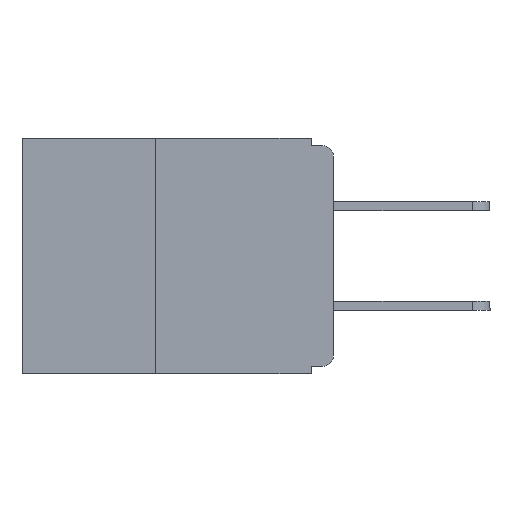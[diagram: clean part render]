
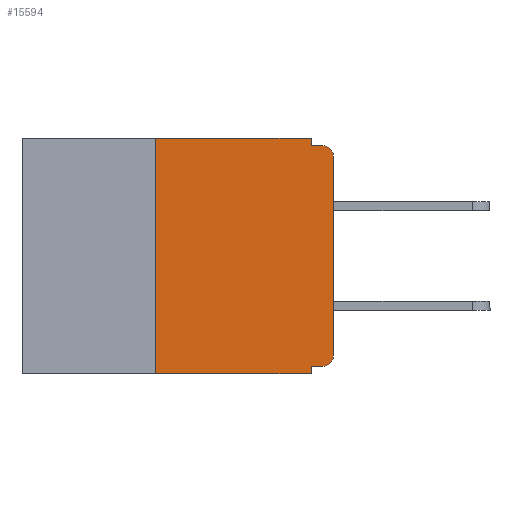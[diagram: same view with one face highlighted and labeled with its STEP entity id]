
A CAD part, left-side view. The second image highlights one B-rep face of the part: STEP entity #15594.
In plain terms, the highlighted planar face has unit normal (-1, 0, 0).
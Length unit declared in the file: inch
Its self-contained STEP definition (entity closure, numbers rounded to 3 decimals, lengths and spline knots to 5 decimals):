
#135 = VECTOR ( 'NONE', #13680, 39.37008 ) ;
#245 = ORIENTED_EDGE ( 'NONE', *, *, #13880, .F. ) ;
#1009 = DIRECTION ( 'NONE',  ( 1., 0., 0. ) ) ;
#1270 = CIRCLE ( 'NONE', #19339, 0.015 ) ;
#1328 = ORIENTED_EDGE ( 'NONE', *, *, #21531, .F. ) ;
#1912 = EDGE_CURVE ( 'NONE', #27886, #9765, #8707, .T. ) ;
#2496 = DIRECTION ( 'NONE',  ( 0., 0., 1. ) ) ;
#3383 = CARTESIAN_POINT ( 'NONE',  ( 0., 0.031, -0.33 ) ) ;
#4471 = ORIENTED_EDGE ( 'NONE', *, *, #13681, .F. ) ;
#4814 = CARTESIAN_POINT ( 'NONE',  ( 0., 0.031, -0.32 ) ) ;
#4955 = CIRCLE ( 'NONE', #18206, 0.015 ) ;
#5346 = ORIENTED_EDGE ( 'NONE', *, *, #5774, .T. ) ;
#5774 = EDGE_CURVE ( 'NONE', #19028, #27886, #1270, .T. ) ;
#6316 = VECTOR ( 'NONE', #6517, 39.37008 ) ;
#6464 = CARTESIAN_POINT ( 'NONE',  ( 0., 0.25, -0.33 ) ) ;
#6517 = DIRECTION ( 'NONE',  ( 0., -1., 0. ) ) ;
#6960 = ORIENTED_EDGE ( 'NONE', *, *, #13703, .F. ) ;
#7206 = VERTEX_POINT ( 'NONE', #22208 ) ;
#8259 = VECTOR ( 'NONE', #17583, 39.37008 ) ;
#8707 = LINE ( 'NONE', #19520, #20483 ) ;
#8971 = EDGE_CURVE ( 'NONE', #9765, #16432, #4955, .T. ) ;
#9235 = FACE_OUTER_BOUND ( 'NONE', #9825, .T. ) ;
#9678 = VECTOR ( 'NONE', #15161, 39.37008 ) ;
#9765 = VERTEX_POINT ( 'NONE', #27728 ) ;
#9825 = EDGE_LOOP ( 'NONE', ( #23399, #10330, #1328, #25685, #4471, #245, #16943, #15319, #6960, #5346 ) ) ;
#9868 = AXIS2_PLACEMENT_3D ( 'NONE', #29062, #1009, #17706 ) ;
#10330 = ORIENTED_EDGE ( 'NONE', *, *, #8971, .T. ) ;
#10779 = EDGE_CURVE ( 'NONE', #22844, #21297, #15906, .T. ) ;
#10891 = VERTEX_POINT ( 'NONE', #13213 ) ;
#11137 = CARTESIAN_POINT ( 'NONE',  ( 0., 0., -0.305 ) ) ;
#11916 = VECTOR ( 'NONE', #29745, 39.37008 ) ;
#12037 = DIRECTION ( 'NONE',  ( -1., 0., 0. ) ) ;
#12038 = CARTESIAN_POINT ( 'NONE',  ( 0., 0.015, -0.32 ) ) ;
#12330 = EDGE_CURVE ( 'NONE', #15108, #21297, #20432, .T. ) ;
#12396 = CARTESIAN_POINT ( 'NONE',  ( 0., 0.25, 0. ) ) ;
#12648 = DIRECTION ( 'NONE',  ( 0., 0., -1. ) ) ;
#12677 = DIRECTION ( 'NONE',  ( -1., 0., 0. ) ) ;
#12928 = LINE ( 'NONE', #27527, #135 ) ;
#12937 = CARTESIAN_POINT ( 'NONE',  ( 0., 0.015, -0.305 ) ) ;
#13213 = CARTESIAN_POINT ( 'NONE',  ( 0., 0.031, 0. ) ) ;
#13680 = DIRECTION ( 'NONE',  ( 0., -1., 0. ) ) ;
#13681 = EDGE_CURVE ( 'NONE', #22950, #10891, #24967, .T. ) ;
#13703 = EDGE_CURVE ( 'NONE', #19028, #22844, #24249, .T. ) ;
#13880 = EDGE_CURVE ( 'NONE', #15108, #22950, #19256, .T. ) ;
#14162 = VECTOR ( 'NONE', #22301, 39.37008 ) ;
#15108 = VERTEX_POINT ( 'NONE', #6464 ) ;
#15161 = DIRECTION ( 'NONE',  ( 0., 0., -1. ) ) ;
#15319 = ORIENTED_EDGE ( 'NONE', *, *, #10779, .F. ) ;
#15594 = ADVANCED_FACE ( 'NONE', ( #9235 ), #26820, .F. ) ;
#15906 = LINE ( 'NONE', #28922, #9678 ) ;
#16432 = VERTEX_POINT ( 'NONE', #23006 ) ;
#16736 = CARTESIAN_POINT ( 'NONE',  ( 0., 0.25, -0.33 ) ) ;
#16943 = ORIENTED_EDGE ( 'NONE', *, *, #12330, .T. ) ;
#17583 = DIRECTION ( 'NONE',  ( 0., 0., -1. ) ) ;
#17706 = DIRECTION ( 'NONE',  ( 0., 0., -1. ) ) ;
#18206 = AXIS2_PLACEMENT_3D ( 'NONE', #25896, #12037, #28182 ) ;
#18639 = EDGE_CURVE ( 'NONE', #10891, #7206, #26828, .T. ) ;
#19028 = VERTEX_POINT ( 'NONE', #12038 ) ;
#19256 = LINE ( 'NONE', #16736, #26029 ) ;
#19339 = AXIS2_PLACEMENT_3D ( 'NONE', #12937, #12677, #12648 ) ;
#19520 = CARTESIAN_POINT ( 'NONE',  ( 0., 0., 0. ) ) ;
#20432 = LINE ( 'NONE', #26775, #14162 ) ;
#20483 = VECTOR ( 'NONE', #30037, 39.37008 ) ;
#20643 = CARTESIAN_POINT ( 'NONE',  ( 0., 0., -0.32 ) ) ;
#21297 = VERTEX_POINT ( 'NONE', #3383 ) ;
#21531 = EDGE_CURVE ( 'NONE', #7206, #16432, #12928, .T. ) ;
#22208 = CARTESIAN_POINT ( 'NONE',  ( 0., 0.031, -0.01 ) ) ;
#22236 = CARTESIAN_POINT ( 'NONE',  ( 0., 0.031, 0. ) ) ;
#22301 = DIRECTION ( 'NONE',  ( 0., -1., 0. ) ) ;
#22844 = VERTEX_POINT ( 'NONE', #4814 ) ;
#22950 = VERTEX_POINT ( 'NONE', #12396 ) ;
#23006 = CARTESIAN_POINT ( 'NONE',  ( 0., 0.015, -0.01 ) ) ;
#23399 = ORIENTED_EDGE ( 'NONE', *, *, #1912, .T. ) ;
#24249 = LINE ( 'NONE', #20643, #11916 ) ;
#24967 = LINE ( 'NONE', #27403, #6316 ) ;
#25685 = ORIENTED_EDGE ( 'NONE', *, *, #18639, .F. ) ;
#25896 = CARTESIAN_POINT ( 'NONE',  ( 0., 0.015, -0.025 ) ) ;
#26029 = VECTOR ( 'NONE', #2496, 39.37008 ) ;
#26775 = CARTESIAN_POINT ( 'NONE',  ( 0., 0.437, -0.33 ) ) ;
#26820 = PLANE ( 'NONE',  #9868 ) ;
#26828 = LINE ( 'NONE', #22236, #8259 ) ;
#27403 = CARTESIAN_POINT ( 'NONE',  ( 0., 0.437, 0. ) ) ;
#27527 = CARTESIAN_POINT ( 'NONE',  ( 0., 0., -0.01 ) ) ;
#27728 = CARTESIAN_POINT ( 'NONE',  ( 0., 0., -0.025 ) ) ;
#27886 = VERTEX_POINT ( 'NONE', #11137 ) ;
#28182 = DIRECTION ( 'NONE',  ( 0., 0., -1. ) ) ;
#28922 = CARTESIAN_POINT ( 'NONE',  ( 0., 0.031, -0.33 ) ) ;
#29062 = CARTESIAN_POINT ( 'NONE',  ( 0., 0.437, 0. ) ) ;
#29745 = DIRECTION ( 'NONE',  ( 0., 1., 0. ) ) ;
#30037 = DIRECTION ( 'NONE',  ( 0., 0., 1. ) ) ;
